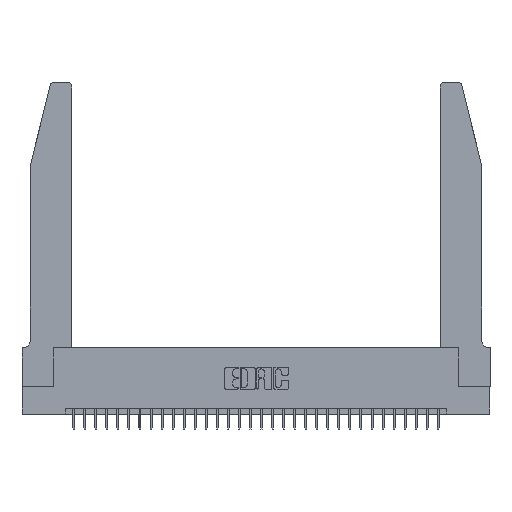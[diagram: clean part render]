
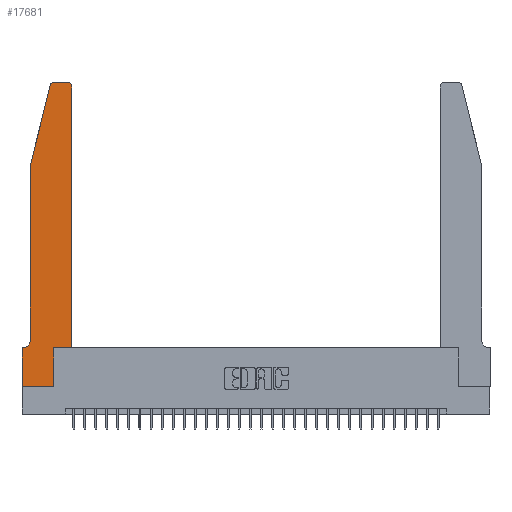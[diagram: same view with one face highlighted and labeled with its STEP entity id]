
A CAD part, top view. The second image highlights one B-rep face of the part: STEP entity #17681.
In plain terms, the highlighted planar face has unit normal (0, 0, 1).
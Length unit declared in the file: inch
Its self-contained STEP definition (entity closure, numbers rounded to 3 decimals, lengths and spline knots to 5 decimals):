
#119 = DIRECTION ( 'NONE',  ( 1., 0., 0. ) ) ;
#336 = LINE ( 'NONE', #23306, #25695 ) ;
#710 = VERTEX_POINT ( 'NONE', #3206 ) ;
#829 = DIRECTION ( 'NONE',  ( -0.239, -0.971, 0. ) ) ;
#1286 = PLANE ( 'NONE',  #19589 ) ;
#1668 = DIRECTION ( 'NONE',  ( 0., 1., 0. ) ) ;
#1669 = EDGE_CURVE ( 'NONE', #22973, #14118, #30736, .T. ) ;
#1878 = VERTEX_POINT ( 'NONE', #12059 ) ;
#2058 = CARTESIAN_POINT ( 'NONE',  ( 0.4505, 2.72, 0.37 ) ) ;
#2982 = EDGE_CURVE ( 'NONE', #20220, #8225, #8245, .T. ) ;
#3206 = CARTESIAN_POINT ( 'NONE',  ( 0.2865, 0.35, 0.37 ) ) ;
#3231 = DIRECTION ( 'NONE',  ( 0., 0., 1. ) ) ;
#3264 = FACE_OUTER_BOUND ( 'NONE', #28849, .T. ) ;
#3506 = CARTESIAN_POINT ( 'NONE',  ( 0., 0.35, 0.37 ) ) ;
#3630 = ORIENTED_EDGE ( 'NONE', *, *, #27474, .T. ) ;
#3991 = ORIENTED_EDGE ( 'NONE', *, *, #8570, .T. ) ;
#3996 = CARTESIAN_POINT ( 'NONE',  ( 0., 0., 0.37 ) ) ;
#4469 = ORIENTED_EDGE ( 'NONE', *, *, #26005, .T. ) ;
#5484 = VECTOR ( 'NONE', #829, 39.37008 ) ;
#5559 = VECTOR ( 'NONE', #13759, 39.37008 ) ;
#6214 = ORIENTED_EDGE ( 'NONE', *, *, #1669, .T. ) ;
#6484 = CARTESIAN_POINT ( 'NONE',  ( 0.4205, 2.75, 0.37 ) ) ;
#6491 = DIRECTION ( 'NONE',  ( 0., -1., 0. ) ) ;
#7012 = CARTESIAN_POINT ( 'NONE',  ( 0.4505, 0.35, 0.37 ) ) ;
#7356 = EDGE_CURVE ( 'NONE', #10519, #20142, #21539, .T. ) ;
#7503 = LINE ( 'NONE', #14483, #17366 ) ;
#7853 = LINE ( 'NONE', #24905, #32436 ) ;
#8219 = DIRECTION ( 'NONE',  ( 0., 0., 1. ) ) ;
#8225 = VERTEX_POINT ( 'NONE', #13531 ) ;
#8245 = LINE ( 'NONE', #8579, #5484 ) ;
#8570 = EDGE_CURVE ( 'NONE', #24105, #10519, #7853, .T. ) ;
#8579 = CARTESIAN_POINT ( 'NONE',  ( 0.0755, 2., 0.37 ) ) ;
#8930 = CARTESIAN_POINT ( 'NONE',  ( 0.2865, 0.35, 0.37 ) ) ;
#10264 = CARTESIAN_POINT ( 'NONE',  ( 0.0055, 0.42, 0.37 ) ) ;
#10519 = VERTEX_POINT ( 'NONE', #3506 ) ;
#10562 = DIRECTION ( 'NONE',  ( 1., 0., 0. ) ) ;
#10725 = ORIENTED_EDGE ( 'NONE', *, *, #31157, .T. ) ;
#11117 = CARTESIAN_POINT ( 'NONE',  ( 0., 0., 0.37 ) ) ;
#12059 = CARTESIAN_POINT ( 'NONE',  ( 0.284, 2.75, 0.37 ) ) ;
#12534 = ORIENTED_EDGE ( 'NONE', *, *, #2982, .T. ) ;
#12882 = CARTESIAN_POINT ( 'NONE',  ( 0.25487, 2.72718, 0.37 ) ) ;
#12987 = AXIS2_PLACEMENT_3D ( 'NONE', #10264, #20852, #20365 ) ;
#13064 = DIRECTION ( 'NONE',  ( 0., -1., 0. ) ) ;
#13333 = DIRECTION ( 'NONE',  ( 1., 0., 0. ) ) ;
#13531 = CARTESIAN_POINT ( 'NONE',  ( 0.0755, 2., 0.37 ) ) ;
#13759 = DIRECTION ( 'NONE',  ( 1., 0., 0. ) ) ;
#14118 = VERTEX_POINT ( 'NONE', #6484 ) ;
#14483 = CARTESIAN_POINT ( 'NONE',  ( 0.2605, 2.75, 0.37 ) ) ;
#15057 = EDGE_CURVE ( 'NONE', #14118, #1878, #7503, .T. ) ;
#15271 = CIRCLE ( 'NONE', #22645, 0.03 ) ;
#16391 = ORIENTED_EDGE ( 'NONE', *, *, #15057, .T. ) ;
#16878 = VECTOR ( 'NONE', #1668, 39.37008 ) ;
#16981 = ORIENTED_EDGE ( 'NONE', *, *, #24763, .T. ) ;
#17111 = DIRECTION ( 'NONE',  ( 0., 1., 0. ) ) ;
#17366 = VECTOR ( 'NONE', #32290, 39.37008 ) ;
#17681 = ADVANCED_FACE ( 'NONE', ( #3264 ), #1286, .T. ) ;
#18180 = CARTESIAN_POINT ( 'NONE',  ( 0.4205, 2.72, 0.37 ) ) ;
#18604 = ORIENTED_EDGE ( 'NONE', *, *, #29083, .T. ) ;
#19025 = LINE ( 'NONE', #8930, #16878 ) ;
#19040 = LINE ( 'NONE', #3996, #5559 ) ;
#19589 = AXIS2_PLACEMENT_3D ( 'NONE', #28873, #8219, #26412 ) ;
#19604 = CARTESIAN_POINT ( 'NONE',  ( 0.0055, 0.35, 0.37 ) ) ;
#20003 = VERTEX_POINT ( 'NONE', #21058 ) ;
#20142 = VERTEX_POINT ( 'NONE', #24628 ) ;
#20220 = VERTEX_POINT ( 'NONE', #12882 ) ;
#20365 = DIRECTION ( 'NONE',  ( -1., 0., 0. ) ) ;
#20852 = DIRECTION ( 'NONE',  ( 0., 0., -1. ) ) ;
#21058 = CARTESIAN_POINT ( 'NONE',  ( 0.4505, 0.35, 0.37 ) ) ;
#21539 = LINE ( 'NONE', #11117, #23442 ) ;
#21710 = CARTESIAN_POINT ( 'NONE',  ( 0.2865, 0., 0.37 ) ) ;
#22162 = ORIENTED_EDGE ( 'NONE', *, *, #7356, .T. ) ;
#22645 = AXIS2_PLACEMENT_3D ( 'NONE', #23402, #3231, #13333 ) ;
#22914 = LINE ( 'NONE', #27861, #32118 ) ;
#22973 = VERTEX_POINT ( 'NONE', #2058 ) ;
#23306 = CARTESIAN_POINT ( 'NONE',  ( 0.0755, 2., 0.37 ) ) ;
#23402 = CARTESIAN_POINT ( 'NONE',  ( 0.284, 2.72, 0.37 ) ) ;
#23442 = VECTOR ( 'NONE', #6491, 39.37008 ) ;
#23629 = ORIENTED_EDGE ( 'NONE', *, *, #30124, .T. ) ;
#24105 = VERTEX_POINT ( 'NONE', #19604 ) ;
#24395 = VERTEX_POINT ( 'NONE', #21710 ) ;
#24628 = CARTESIAN_POINT ( 'NONE',  ( 0., 0., 0.37 ) ) ;
#24763 = EDGE_CURVE ( 'NONE', #32577, #24105, #25099, .T. ) ;
#24783 = CARTESIAN_POINT ( 'NONE',  ( 0.0755, 0.42, 0.37 ) ) ;
#24905 = CARTESIAN_POINT ( 'NONE',  ( 0.0755, 0.35, 0.37 ) ) ;
#25099 = CIRCLE ( 'NONE', #12987, 0.07 ) ;
#25495 = AXIS2_PLACEMENT_3D ( 'NONE', #18180, #28087, #10562 ) ;
#25695 = VECTOR ( 'NONE', #13064, 39.37008 ) ;
#26005 = EDGE_CURVE ( 'NONE', #20142, #24395, #19040, .T. ) ;
#26412 = DIRECTION ( 'NONE',  ( 1., 0., 0. ) ) ;
#26836 = VECTOR ( 'NONE', #17111, 39.37008 ) ;
#27474 = EDGE_CURVE ( 'NONE', #8225, #32577, #336, .T. ) ;
#27708 = DIRECTION ( 'NONE',  ( -1., 0., 0. ) ) ;
#27861 = CARTESIAN_POINT ( 'NONE',  ( 0.4505, 0.35, 0.37 ) ) ;
#28087 = DIRECTION ( 'NONE',  ( 0., 0., 1. ) ) ;
#28849 = EDGE_LOOP ( 'NONE', ( #16391, #30665, #12534, #3630, #16981, #3991, #22162, #4469, #10725, #23629, #18604, #6214 ) ) ;
#28873 = CARTESIAN_POINT ( 'NONE',  ( 0., 0.35, 0.37 ) ) ;
#29083 = EDGE_CURVE ( 'NONE', #20003, #22973, #29650, .T. ) ;
#29650 = LINE ( 'NONE', #7012, #26836 ) ;
#30124 = EDGE_CURVE ( 'NONE', #710, #20003, #22914, .T. ) ;
#30408 = EDGE_CURVE ( 'NONE', #1878, #20220, #15271, .T. ) ;
#30665 = ORIENTED_EDGE ( 'NONE', *, *, #30408, .T. ) ;
#30736 = CIRCLE ( 'NONE', #25495, 0.03 ) ;
#31157 = EDGE_CURVE ( 'NONE', #24395, #710, #19025, .T. ) ;
#32118 = VECTOR ( 'NONE', #119, 39.37008 ) ;
#32290 = DIRECTION ( 'NONE',  ( -1., 0., 0. ) ) ;
#32436 = VECTOR ( 'NONE', #27708, 39.37008 ) ;
#32577 = VERTEX_POINT ( 'NONE', #24783 ) ;
